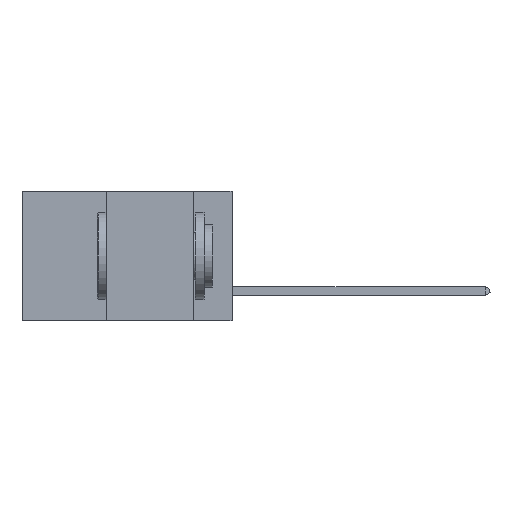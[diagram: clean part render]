
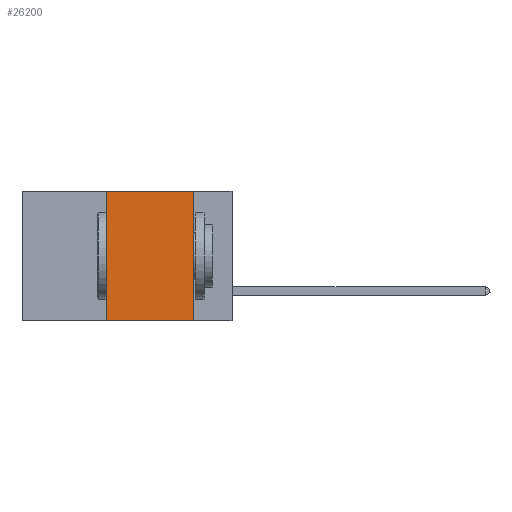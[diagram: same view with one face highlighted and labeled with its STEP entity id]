
A CAD part, left-side view. The second image highlights one B-rep face of the part: STEP entity #26200.
In plain terms, the highlighted planar face has unit normal (-1, 0, 0).
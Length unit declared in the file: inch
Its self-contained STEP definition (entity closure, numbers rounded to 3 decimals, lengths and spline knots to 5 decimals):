
#486 = CARTESIAN_POINT ( 'NONE',  ( 0., 0.36, 0. ) ) ;
#878 = CARTESIAN_POINT ( 'NONE',  ( 0., 0.36, 0. ) ) ;
#3980 = PLANE ( 'NONE',  #34337 ) ;
#4528 = VECTOR ( 'NONE', #25886, 39.37008 ) ;
#5117 = ORIENTED_EDGE ( 'NONE', *, *, #20856, .F. ) ;
#7428 = CARTESIAN_POINT ( 'NONE',  ( 0., 0.6, 0. ) ) ;
#7461 = LINE ( 'NONE', #13733, #24197 ) ;
#11560 = EDGE_CURVE ( 'NONE', #28841, #12562, #22387, .T. ) ;
#12562 = VERTEX_POINT ( 'NONE', #486 ) ;
#13733 = CARTESIAN_POINT ( 'NONE',  ( 0., 0.6, -0.37 ) ) ;
#13902 = DIRECTION ( 'NONE',  ( 0., 0., -1. ) ) ;
#14344 = EDGE_LOOP ( 'NONE', ( #27530, #5117, #17271, #44961 ) ) ;
#14933 = DIRECTION ( 'NONE',  ( 0., -1., 0. ) ) ;
#15046 = DIRECTION ( 'NONE',  ( 0., -1., 0. ) ) ;
#16249 = CARTESIAN_POINT ( 'NONE',  ( 0., 0.36, -0.37 ) ) ;
#17271 = ORIENTED_EDGE ( 'NONE', *, *, #11560, .F. ) ;
#17703 = EDGE_CURVE ( 'NONE', #44238, #34182, #30426, .T. ) ;
#18006 = CARTESIAN_POINT ( 'NONE',  ( 0., 0.6, 0. ) ) ;
#20856 = EDGE_CURVE ( 'NONE', #12562, #44238, #31348, .T. ) ;
#21230 = CARTESIAN_POINT ( 'NONE',  ( 0., 0.11, 0. ) ) ;
#22387 = LINE ( 'NONE', #878, #4528 ) ;
#24197 = VECTOR ( 'NONE', #14933, 39.37008 ) ;
#25886 = DIRECTION ( 'NONE',  ( 0., 0., 1. ) ) ;
#26200 = ADVANCED_FACE ( 'NONE', ( #33869 ), #3980, .F. ) ;
#27530 = ORIENTED_EDGE ( 'NONE', *, *, #17703, .F. ) ;
#28570 = VECTOR ( 'NONE', #15046, 39.37008 ) ;
#28841 = VERTEX_POINT ( 'NONE', #16249 ) ;
#30426 = LINE ( 'NONE', #21230, #32135 ) ;
#31348 = LINE ( 'NONE', #7428, #28570 ) ;
#32135 = VECTOR ( 'NONE', #13902, 39.37008 ) ;
#33869 = FACE_OUTER_BOUND ( 'NONE', #14344, .T. ) ;
#34182 = VERTEX_POINT ( 'NONE', #41243 ) ;
#34337 = AXIS2_PLACEMENT_3D ( 'NONE', #18006, #39794, #39646 ) ;
#34987 = CARTESIAN_POINT ( 'NONE',  ( 0., 0.11, 0. ) ) ;
#39646 = DIRECTION ( 'NONE',  ( 0., 0., -1. ) ) ;
#39794 = DIRECTION ( 'NONE',  ( 1., 0., 0. ) ) ;
#41243 = CARTESIAN_POINT ( 'NONE',  ( 0., 0.11, -0.37 ) ) ;
#42603 = EDGE_CURVE ( 'NONE', #28841, #34182, #7461, .T. ) ;
#44238 = VERTEX_POINT ( 'NONE', #34987 ) ;
#44961 = ORIENTED_EDGE ( 'NONE', *, *, #42603, .T. ) ;
